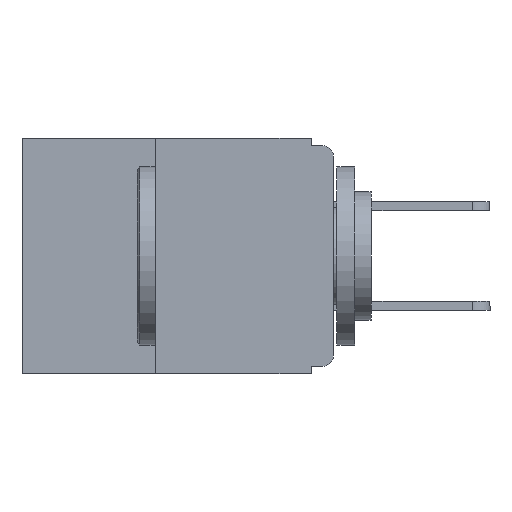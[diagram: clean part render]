
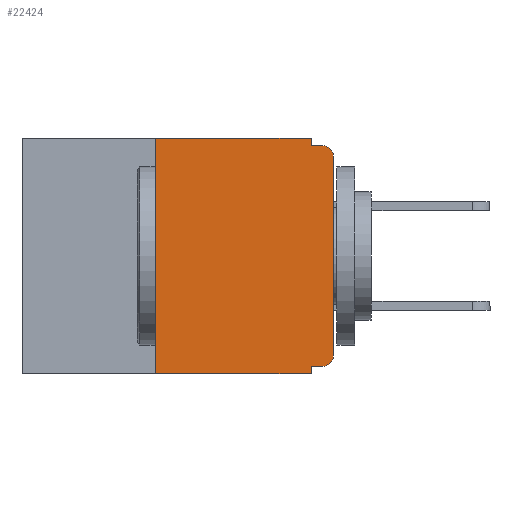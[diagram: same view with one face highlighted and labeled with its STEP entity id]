
A CAD part, left-side view. The second image highlights one B-rep face of the part: STEP entity #22424.
In plain terms, the highlighted planar face has unit normal (-1, 0, 0).
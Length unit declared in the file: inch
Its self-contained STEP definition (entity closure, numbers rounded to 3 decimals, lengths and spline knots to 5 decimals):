
#270 = CARTESIAN_POINT ( 'NONE',  ( 0., 0.031, -0.32 ) ) ;
#1250 = EDGE_CURVE ( 'NONE', #12508, #13405, #14325, .T. ) ;
#1396 = ORIENTED_EDGE ( 'NONE', *, *, #10247, .T. ) ;
#1559 = ORIENTED_EDGE ( 'NONE', *, *, #5959, .T. ) ;
#1648 = VERTEX_POINT ( 'NONE', #17707 ) ;
#1776 = CARTESIAN_POINT ( 'NONE',  ( 0., 0.015, -0.305 ) ) ;
#2022 = ORIENTED_EDGE ( 'NONE', *, *, #2867, .F. ) ;
#2318 = CARTESIAN_POINT ( 'NONE',  ( 0., 0.015, -0.32 ) ) ;
#2514 = VECTOR ( 'NONE', #26316, 39.37008 ) ;
#2707 = ORIENTED_EDGE ( 'NONE', *, *, #9990, .F. ) ;
#2867 = EDGE_CURVE ( 'NONE', #3364, #7746, #19759, .T. ) ;
#3328 = ORIENTED_EDGE ( 'NONE', *, *, #24036, .F. ) ;
#3364 = VERTEX_POINT ( 'NONE', #22613 ) ;
#3736 = ORIENTED_EDGE ( 'NONE', *, *, #4598, .F. ) ;
#4598 = EDGE_CURVE ( 'NONE', #12799, #13411, #20726, .T. ) ;
#4727 = ORIENTED_EDGE ( 'NONE', *, *, #19436, .T. ) ;
#4804 = ORIENTED_EDGE ( 'NONE', *, *, #21123, .F. ) ;
#5169 = ORIENTED_EDGE ( 'NONE', *, *, #13282, .F. ) ;
#5378 = LINE ( 'NONE', #15098, #27774 ) ;
#5959 = EDGE_CURVE ( 'NONE', #18494, #7746, #20393, .T. ) ;
#6228 = ORIENTED_EDGE ( 'NONE', *, *, #1250, .T. ) ;
#7543 = DIRECTION ( 'NONE',  ( 0., 1., 0. ) ) ;
#7652 = CARTESIAN_POINT ( 'NONE',  ( 0., 0., -0.025 ) ) ;
#7746 = VERTEX_POINT ( 'NONE', #10762 ) ;
#8182 = DIRECTION ( 'NONE',  ( 1., 0., 0. ) ) ;
#8943 = CARTESIAN_POINT ( 'NONE',  ( 0., 0.031, -0.33 ) ) ;
#9990 = EDGE_CURVE ( 'NONE', #1648, #3364, #27878, .T. ) ;
#10046 = DIRECTION ( 'NONE',  ( 0., 0., -1. ) ) ;
#10228 = LINE ( 'NONE', #22610, #26900 ) ;
#10247 = EDGE_CURVE ( 'NONE', #13405, #18494, #10228, .T. ) ;
#10257 = PLANE ( 'NONE',  #27386 ) ;
#10432 = VECTOR ( 'NONE', #17630, 39.37008 ) ;
#10762 = CARTESIAN_POINT ( 'NONE',  ( 0., 0.015, -0.01 ) ) ;
#10844 = DIRECTION ( 'NONE',  ( 0., 0., -1. ) ) ;
#12458 = DIRECTION ( 'NONE',  ( -1., 0., 0. ) ) ;
#12508 = VERTEX_POINT ( 'NONE', #2318 ) ;
#12799 = VERTEX_POINT ( 'NONE', #22916 ) ;
#13236 = CARTESIAN_POINT ( 'NONE',  ( 0., 0.437, 0. ) ) ;
#13282 = EDGE_CURVE ( 'NONE', #12508, #15597, #14666, .T. ) ;
#13405 = VERTEX_POINT ( 'NONE', #25350 ) ;
#13411 = VERTEX_POINT ( 'NONE', #18892 ) ;
#13979 = VECTOR ( 'NONE', #7543, 39.37008 ) ;
#14149 = EDGE_LOOP ( 'NONE', ( #1396, #1559, #2022, #2707, #3328, #3736, #4727, #4804, #5169, #6228 ) ) ;
#14182 = AXIS2_PLACEMENT_3D ( 'NONE', #18442, #18498, #18439 ) ;
#14325 = CIRCLE ( 'NONE', #25778, 0.015 ) ;
#14666 = LINE ( 'NONE', #20527, #13979 ) ;
#14847 = VECTOR ( 'NONE', #10046, 39.37008 ) ;
#15098 = CARTESIAN_POINT ( 'NONE',  ( 0., 0.437, -0.33 ) ) ;
#15597 = VERTEX_POINT ( 'NONE', #270 ) ;
#15880 = DIRECTION ( 'NONE',  ( 0., 0., 1. ) ) ;
#17630 = DIRECTION ( 'NONE',  ( 0., 0., 1. ) ) ;
#17700 = CARTESIAN_POINT ( 'NONE',  ( 0., 0.25, -0.33 ) ) ;
#17707 = CARTESIAN_POINT ( 'NONE',  ( 0., 0.031, 0. ) ) ;
#18439 = DIRECTION ( 'NONE',  ( 0., 0., -1. ) ) ;
#18442 = CARTESIAN_POINT ( 'NONE',  ( 0., 0.015, -0.025 ) ) ;
#18494 = VERTEX_POINT ( 'NONE', #7652 ) ;
#18498 = DIRECTION ( 'NONE',  ( -1., 0., 0. ) ) ;
#18892 = CARTESIAN_POINT ( 'NONE',  ( 0., 0.25, 0. ) ) ;
#18929 = VERTEX_POINT ( 'NONE', #8943 ) ;
#19072 = CARTESIAN_POINT ( 'NONE',  ( 0., 0.437, 0. ) ) ;
#19436 = EDGE_CURVE ( 'NONE', #12799, #18929, #5378, .T. ) ;
#19563 = CARTESIAN_POINT ( 'NONE',  ( 0., 0.031, 0. ) ) ;
#19759 = LINE ( 'NONE', #20924, #26832 ) ;
#19941 = LINE ( 'NONE', #13236, #2514 ) ;
#20393 = CIRCLE ( 'NONE', #14182, 0.015 ) ;
#20414 = DIRECTION ( 'NONE',  ( 0., -1., 0. ) ) ;
#20527 = CARTESIAN_POINT ( 'NONE',  ( 0., 0., -0.32 ) ) ;
#20726 = LINE ( 'NONE', #17700, #10432 ) ;
#20924 = CARTESIAN_POINT ( 'NONE',  ( 0., 0., -0.01 ) ) ;
#20980 = CARTESIAN_POINT ( 'NONE',  ( 0., 0.031, -0.33 ) ) ;
#21123 = EDGE_CURVE ( 'NONE', #15597, #18929, #26440, .T. ) ;
#21323 = FACE_OUTER_BOUND ( 'NONE', #14149, .T. ) ;
#21843 = DIRECTION ( 'NONE',  ( 0., -1., 0. ) ) ;
#22121 = DIRECTION ( 'NONE',  ( 0., 0., -1. ) ) ;
#22253 = VECTOR ( 'NONE', #10844, 39.37008 ) ;
#22424 = ADVANCED_FACE ( 'NONE', ( #21323 ), #10257, .F. ) ;
#22610 = CARTESIAN_POINT ( 'NONE',  ( 0., 0., 0. ) ) ;
#22613 = CARTESIAN_POINT ( 'NONE',  ( 0., 0.031, -0.01 ) ) ;
#22916 = CARTESIAN_POINT ( 'NONE',  ( 0., 0.25, -0.33 ) ) ;
#23440 = DIRECTION ( 'NONE',  ( 0., 0., -1. ) ) ;
#24036 = EDGE_CURVE ( 'NONE', #13411, #1648, #19941, .T. ) ;
#25350 = CARTESIAN_POINT ( 'NONE',  ( 0., 0., -0.305 ) ) ;
#25778 = AXIS2_PLACEMENT_3D ( 'NONE', #1776, #12458, #22121 ) ;
#26316 = DIRECTION ( 'NONE',  ( 0., -1., 0. ) ) ;
#26440 = LINE ( 'NONE', #20980, #14847 ) ;
#26832 = VECTOR ( 'NONE', #20414, 39.37008 ) ;
#26900 = VECTOR ( 'NONE', #15880, 39.37008 ) ;
#27386 = AXIS2_PLACEMENT_3D ( 'NONE', #19072, #8182, #23440 ) ;
#27774 = VECTOR ( 'NONE', #21843, 39.37008 ) ;
#27878 = LINE ( 'NONE', #19563, #22253 ) ;
